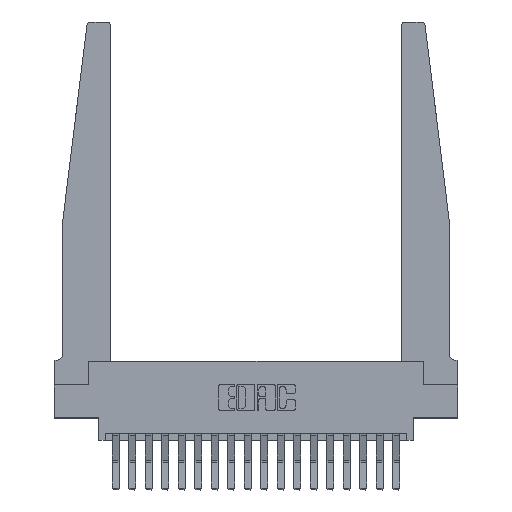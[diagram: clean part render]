
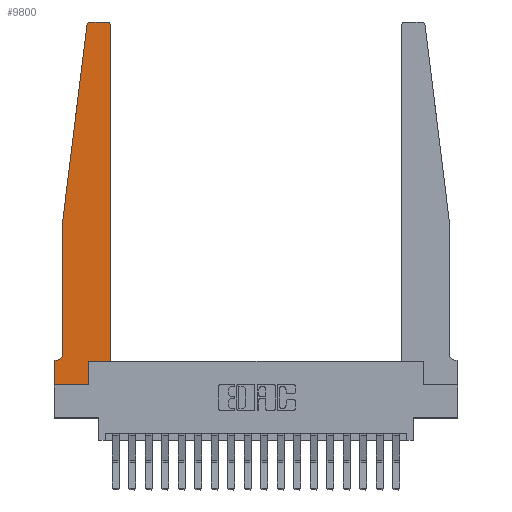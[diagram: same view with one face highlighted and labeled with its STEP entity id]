
A CAD part, top view. The second image highlights one B-rep face of the part: STEP entity #9800.
In plain terms, the highlighted planar face has unit normal (0, 0, 1).
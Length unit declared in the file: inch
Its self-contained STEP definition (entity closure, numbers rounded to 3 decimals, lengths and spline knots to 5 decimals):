
#200 = VECTOR ( 'NONE', #11045, 39.37008 ) ;
#407 = LINE ( 'NONE', #9793, #7681 ) ;
#685 = CARTESIAN_POINT ( 'NONE',  ( 0.27653, 2.75, 0.37 ) ) ;
#859 = CARTESIAN_POINT ( 'NONE',  ( 0.425, 2.72, 0.37 ) ) ;
#1181 = PLANE ( 'NONE',  #2526 ) ;
#1478 = DIRECTION ( 'NONE',  ( -0.122, -0.992, 0. ) ) ;
#1547 = CARTESIAN_POINT ( 'NONE',  ( 0.2605, 0., 0.37 ) ) ;
#1825 = DIRECTION ( 'NONE',  ( 0., -1., 0. ) ) ;
#2022 = DIRECTION ( 'NONE',  ( 1., 0., 0. ) ) ;
#2526 = AXIS2_PLACEMENT_3D ( 'NONE', #18739, #20269, #7463 ) ;
#2541 = CIRCLE ( 'NONE', #16429, 0.03 ) ;
#2565 = CARTESIAN_POINT ( 'NONE',  ( 0.065, 1.25, 0.37 ) ) ;
#2756 = CARTESIAN_POINT ( 'NONE',  ( 0., 0., 0.37 ) ) ;
#2847 = CARTESIAN_POINT ( 'NONE',  ( 0., 0., 0.37 ) ) ;
#3041 = ORIENTED_EDGE ( 'NONE', *, *, #4348, .T. ) ;
#3797 = LINE ( 'NONE', #10089, #7041 ) ;
#4187 = DIRECTION ( 'NONE',  ( 0., -1., 0. ) ) ;
#4190 = VECTOR ( 'NONE', #7147, 39.37008 ) ;
#4306 = ORIENTED_EDGE ( 'NONE', *, *, #11291, .T. ) ;
#4348 = EDGE_CURVE ( 'NONE', #13992, #4520, #407, .T. ) ;
#4520 = VERTEX_POINT ( 'NONE', #1547 ) ;
#4605 = ORIENTED_EDGE ( 'NONE', *, *, #11040, .T. ) ;
#4858 = CARTESIAN_POINT ( 'NONE',  ( 0.27653, 2.72, 0.37 ) ) ;
#4880 = EDGE_CURVE ( 'NONE', #19823, #7920, #9847, .T. ) ;
#5137 = VECTOR ( 'NONE', #12480, 39.37008 ) ;
#5186 = VERTEX_POINT ( 'NONE', #13609 ) ;
#5395 = ORIENTED_EDGE ( 'NONE', *, *, #13631, .T. ) ;
#5433 = ORIENTED_EDGE ( 'NONE', *, *, #16152, .T. ) ;
#5661 = VERTEX_POINT ( 'NONE', #2565 ) ;
#5973 = CARTESIAN_POINT ( 'NONE',  ( 0.425, 0.18, 0.37 ) ) ;
#6063 = EDGE_CURVE ( 'NONE', #8380, #15893, #6349, .T. ) ;
#6106 = LINE ( 'NONE', #13490, #14425 ) ;
#6349 = CIRCLE ( 'NONE', #17966, 0.03 ) ;
#6498 = VERTEX_POINT ( 'NONE', #19398 ) ;
#6702 = CARTESIAN_POINT ( 'NONE',  ( 0.395, 2.72, 0.37 ) ) ;
#6703 = DIRECTION ( 'NONE',  ( 1., 0., 0. ) ) ;
#6712 = EDGE_CURVE ( 'NONE', #5661, #6498, #3797, .T. ) ;
#6738 = DIRECTION ( 'NONE',  ( -1., 0., 0. ) ) ;
#7041 = VECTOR ( 'NONE', #1825, 39.37008 ) ;
#7147 = DIRECTION ( 'NONE',  ( -1., 0., 0. ) ) ;
#7384 = LINE ( 'NONE', #2756, #20402 ) ;
#7463 = DIRECTION ( 'NONE',  ( 1., 0., 0. ) ) ;
#7681 = VECTOR ( 'NONE', #6703, 39.37008 ) ;
#7920 = VERTEX_POINT ( 'NONE', #9043 ) ;
#8192 = CARTESIAN_POINT ( 'NONE',  ( 0.2605, 0.18, 0.37 ) ) ;
#8380 = VERTEX_POINT ( 'NONE', #685 ) ;
#9043 = CARTESIAN_POINT ( 'NONE',  ( 0.425, 0.18, 0.37 ) ) ;
#9301 = LINE ( 'NONE', #5973, #5137 ) ;
#9445 = ORIENTED_EDGE ( 'NONE', *, *, #15926, .T. ) ;
#9765 = CIRCLE ( 'NONE', #18392, 0.05 ) ;
#9793 = CARTESIAN_POINT ( 'NONE',  ( 0., 0., 0.37 ) ) ;
#9800 = ADVANCED_FACE ( 'NONE', ( #15345 ), #1181, .T. ) ;
#9847 = LINE ( 'NONE', #16199, #18928 ) ;
#10089 = CARTESIAN_POINT ( 'NONE',  ( 0.065, 1.25, 0.37 ) ) ;
#10099 = EDGE_CURVE ( 'NONE', #7920, #14274, #9301, .T. ) ;
#10139 = ORIENTED_EDGE ( 'NONE', *, *, #17877, .T. ) ;
#10471 = ORIENTED_EDGE ( 'NONE', *, *, #15044, .T. ) ;
#11003 = CARTESIAN_POINT ( 'NONE',  ( 0.015, 0.1875, 0.37 ) ) ;
#11040 = EDGE_CURVE ( 'NONE', #15893, #5661, #6106, .T. ) ;
#11045 = DIRECTION ( 'NONE',  ( -1., 0., 0. ) ) ;
#11198 = CARTESIAN_POINT ( 'NONE',  ( 0.015, 0.2375, 0.37 ) ) ;
#11291 = EDGE_CURVE ( 'NONE', #17236, #5186, #11893, .T. ) ;
#11393 = DIRECTION ( 'NONE',  ( 0., 0., -1. ) ) ;
#11456 = DIRECTION ( 'NONE',  ( 0., 0., 1. ) ) ;
#11483 = DIRECTION ( 'NONE',  ( 0., 0., 1. ) ) ;
#11570 = VERTEX_POINT ( 'NONE', #13413 ) ;
#11630 = DIRECTION ( 'NONE',  ( 0., 1., 0. ) ) ;
#11774 = CARTESIAN_POINT ( 'NONE',  ( 0.2605, 0.18, 0.37 ) ) ;
#11893 = LINE ( 'NONE', #19863, #4190 ) ;
#12480 = DIRECTION ( 'NONE',  ( 0., 1., 0. ) ) ;
#13413 = CARTESIAN_POINT ( 'NONE',  ( 0.395, 2.75, 0.37 ) ) ;
#13490 = CARTESIAN_POINT ( 'NONE',  ( 0.065, 1.25, 0.37 ) ) ;
#13609 = CARTESIAN_POINT ( 'NONE',  ( 0., 0.1875, 0.37 ) ) ;
#13631 = EDGE_CURVE ( 'NONE', #4520, #19823, #14531, .T. ) ;
#13684 = ORIENTED_EDGE ( 'NONE', *, *, #10099, .T. ) ;
#13992 = VERTEX_POINT ( 'NONE', #2847 ) ;
#14274 = VERTEX_POINT ( 'NONE', #859 ) ;
#14425 = VECTOR ( 'NONE', #1478, 39.37008 ) ;
#14463 = DIRECTION ( 'NONE',  ( 1., 0., 0. ) ) ;
#14531 = LINE ( 'NONE', #8192, #19403 ) ;
#15044 = EDGE_CURVE ( 'NONE', #5186, #13992, #7384, .T. ) ;
#15166 = ORIENTED_EDGE ( 'NONE', *, *, #6063, .T. ) ;
#15317 = CARTESIAN_POINT ( 'NONE',  ( 0.24675, 2.72367, 0.37 ) ) ;
#15345 = FACE_OUTER_BOUND ( 'NONE', #18688, .T. ) ;
#15893 = VERTEX_POINT ( 'NONE', #15317 ) ;
#15926 = EDGE_CURVE ( 'NONE', #11570, #8380, #18238, .T. ) ;
#16152 = EDGE_CURVE ( 'NONE', #14274, #11570, #2541, .T. ) ;
#16174 = DIRECTION ( 'NONE',  ( 1., 0., 0. ) ) ;
#16199 = CARTESIAN_POINT ( 'NONE',  ( 0.425, 0.18, 0.37 ) ) ;
#16429 = AXIS2_PLACEMENT_3D ( 'NONE', #6702, #11456, #14463 ) ;
#17236 = VERTEX_POINT ( 'NONE', #11003 ) ;
#17877 = EDGE_CURVE ( 'NONE', #6498, #17236, #9765, .T. ) ;
#17966 = AXIS2_PLACEMENT_3D ( 'NONE', #4858, #11483, #16174 ) ;
#18238 = LINE ( 'NONE', #18812, #200 ) ;
#18369 = ORIENTED_EDGE ( 'NONE', *, *, #6712, .T. ) ;
#18392 = AXIS2_PLACEMENT_3D ( 'NONE', #11198, #11393, #6738 ) ;
#18688 = EDGE_LOOP ( 'NONE', ( #9445, #15166, #4605, #18369, #10139, #4306, #10471, #3041, #5395, #19416, #13684, #5433 ) ) ;
#18739 = CARTESIAN_POINT ( 'NONE',  ( 0., 0.1875, 0.37 ) ) ;
#18812 = CARTESIAN_POINT ( 'NONE',  ( 0.25, 2.75, 0.37 ) ) ;
#18928 = VECTOR ( 'NONE', #2022, 39.37008 ) ;
#19398 = CARTESIAN_POINT ( 'NONE',  ( 0.065, 0.2375, 0.37 ) ) ;
#19403 = VECTOR ( 'NONE', #11630, 39.37008 ) ;
#19416 = ORIENTED_EDGE ( 'NONE', *, *, #4880, .T. ) ;
#19823 = VERTEX_POINT ( 'NONE', #11774 ) ;
#19863 = CARTESIAN_POINT ( 'NONE',  ( 0.065, 0.1875, 0.37 ) ) ;
#20269 = DIRECTION ( 'NONE',  ( 0., 0., 1. ) ) ;
#20402 = VECTOR ( 'NONE', #4187, 39.37008 ) ;
